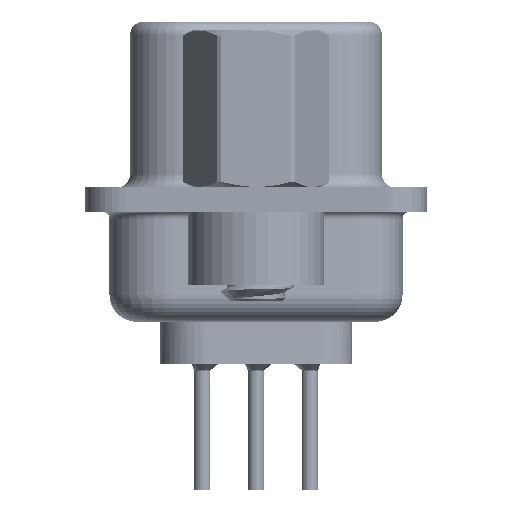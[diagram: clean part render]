
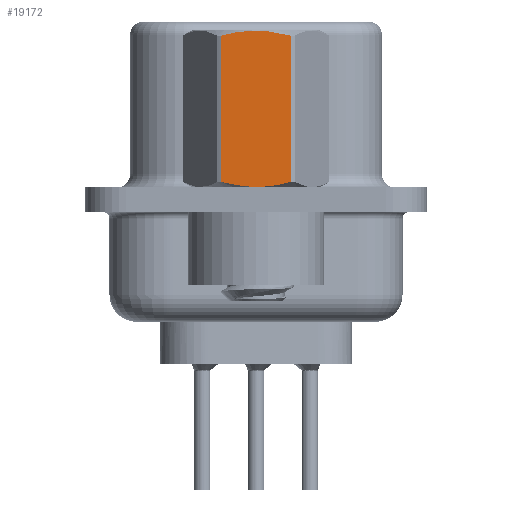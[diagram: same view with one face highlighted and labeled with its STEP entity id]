
A CAD part, left-side view. The second image highlights one B-rep face of the part: STEP entity #19172.
In plain terms, the highlighted planar face has unit normal (-1, 0, 0).
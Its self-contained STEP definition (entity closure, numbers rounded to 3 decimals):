
#540 = ORIENTED_EDGE ( 'NONE', *, *, #24735, .T. ) ;
#886 = CARTESIAN_POINT ( 'NONE',  ( -2.381, -1.273, 0.652 ) ) ;
#1144 = EDGE_CURVE ( 'NONE', #12204, #4828, #18785, .T. ) ;
#1241 = CARTESIAN_POINT ( 'NONE',  ( -2.381, -1.273, 6.048 ) ) ;
#1562 = EDGE_LOOP ( 'NONE', ( #9851, #540, #18021, #11248 ) ) ;
#2813 = DIRECTION ( 'NONE',  ( 0., -1., 0. ) ) ;
#3135 = FACE_OUTER_BOUND ( 'NONE', #1562, .T. ) ;
#3341 = CARTESIAN_POINT ( 'NONE',  ( -2.381, -0.432, 0.485 ) ) ;
#3925 = B_SPLINE_CURVE_WITH_KNOTS ( 'NONE', 3,
 ( #19047, #4468, #31296, #16925, #16293, #14456, #21178, #11202, #26233, #26385 ),
 .UNSPECIFIED., .F., .F.,
 ( 4, 2, 2, 2, 4 ),
 ( 0.001, 0.002, 0.002, 0.003, 0.004 ),
 .UNSPECIFIED. ) ;
#4468 = CARTESIAN_POINT ( 'NONE',  ( -2.381, -1.066, 6.104 ) ) ;
#4522 = VECTOR ( 'NONE', #31127, 1000. ) ;
#4828 = VERTEX_POINT ( 'NONE', #10542 ) ;
#5424 = CARTESIAN_POINT ( 'NONE',  ( -2.381, -1.273, 3.792 ) ) ;
#5780 = CARTESIAN_POINT ( 'NONE',  ( -2.381, 1.273, 0.652 ) ) ;
#6273 = LINE ( 'NONE', #26706, #4522 ) ;
#7728 = DIRECTION ( 'NONE',  ( 0., 0., 1. ) ) ;
#7738 = VERTEX_POINT ( 'NONE', #1241 ) ;
#8043 = CARTESIAN_POINT ( 'NONE',  ( -2.381, 1.375, -3.75 ) ) ;
#9851 = ORIENTED_EDGE ( 'NONE', *, *, #1144, .T. ) ;
#10542 = CARTESIAN_POINT ( 'NONE',  ( -2.381, -1.273, 0.652 ) ) ;
#11202 = CARTESIAN_POINT ( 'NONE',  ( -2.381, 0.853, 6.151 ) ) ;
#11248 = ORIENTED_EDGE ( 'NONE', *, *, #26148, .T. ) ;
#12204 = VERTEX_POINT ( 'NONE', #21133 ) ;
#12988 = CARTESIAN_POINT ( 'NONE',  ( -2.381, 0.428, 0.485 ) ) ;
#13179 = EDGE_CURVE ( 'NONE', #7738, #19596, #3925, .T. ) ;
#13311 = CARTESIAN_POINT ( 'NONE',  ( -2.381, -0.858, 0.55 ) ) ;
#14456 = CARTESIAN_POINT ( 'NONE',  ( -2.381, 0.215, 6.232 ) ) ;
#16293 = CARTESIAN_POINT ( 'NONE',  ( -2.381, -0.215, 6.232 ) ) ;
#16903 = AXIS2_PLACEMENT_3D ( 'NONE', #8043, #20150, #2813 ) ;
#16925 = CARTESIAN_POINT ( 'NONE',  ( -2.381, -0.432, 6.215 ) ) ;
#18021 = ORIENTED_EDGE ( 'NONE', *, *, #13179, .T. ) ;
#18231 = CARTESIAN_POINT ( 'NONE',  ( -2.381, 1.065, 0.596 ) ) ;
#18785 = B_SPLINE_CURVE_WITH_KNOTS ( 'NONE', 3,
 ( #5780, #18231, #28189, #12988, #20684, #25723, #3341, #13311, #23302, #886 ),
 .UNSPECIFIED., .F., .F.,
 ( 4, 2, 2, 2, 4 ),
 ( 0.003, 0.003, 0.004, 0.004, 0.005 ),
 .UNSPECIFIED. ) ;
#19047 = CARTESIAN_POINT ( 'NONE',  ( -2.381, -1.273, 6.048 ) ) ;
#19172 = ADVANCED_FACE ( 'NONE', ( #3135 ), #24880, .T. ) ;
#19596 = VERTEX_POINT ( 'NONE', #22693 ) ;
#20150 = DIRECTION ( 'NONE',  ( -1., 0., 0. ) ) ;
#20684 = CARTESIAN_POINT ( 'NONE',  ( -2.381, 0.215, 0.468 ) ) ;
#21133 = CARTESIAN_POINT ( 'NONE',  ( -2.381, 1.273, 0.652 ) ) ;
#21178 = CARTESIAN_POINT ( 'NONE',  ( -2.381, 0.428, 6.215 ) ) ;
#22693 = CARTESIAN_POINT ( 'NONE',  ( -2.381, 1.273, 6.048 ) ) ;
#23302 = CARTESIAN_POINT ( 'NONE',  ( -2.381, -1.066, 0.596 ) ) ;
#24735 = EDGE_CURVE ( 'NONE', #4828, #7738, #27827, .T. ) ;
#24880 = PLANE ( 'NONE',  #16903 ) ;
#25723 = CARTESIAN_POINT ( 'NONE',  ( -2.381, -0.215, 0.468 ) ) ;
#26148 = EDGE_CURVE ( 'NONE', #19596, #12204, #6273, .T. ) ;
#26233 = CARTESIAN_POINT ( 'NONE',  ( -2.381, 1.065, 6.104 ) ) ;
#26385 = CARTESIAN_POINT ( 'NONE',  ( -2.381, 1.273, 6.048 ) ) ;
#26706 = CARTESIAN_POINT ( 'NONE',  ( -2.381, 1.273, 3.792 ) ) ;
#27827 = LINE ( 'NONE', #5424, #32206 ) ;
#28189 = CARTESIAN_POINT ( 'NONE',  ( -2.381, 0.853, 0.549 ) ) ;
#31127 = DIRECTION ( 'NONE',  ( 0., 0., -1. ) ) ;
#31296 = CARTESIAN_POINT ( 'NONE',  ( -2.381, -0.858, 6.15 ) ) ;
#32206 = VECTOR ( 'NONE', #7728, 1000. ) ;
